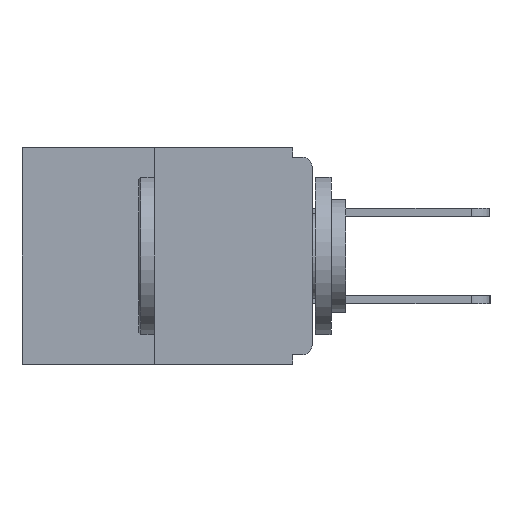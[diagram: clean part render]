
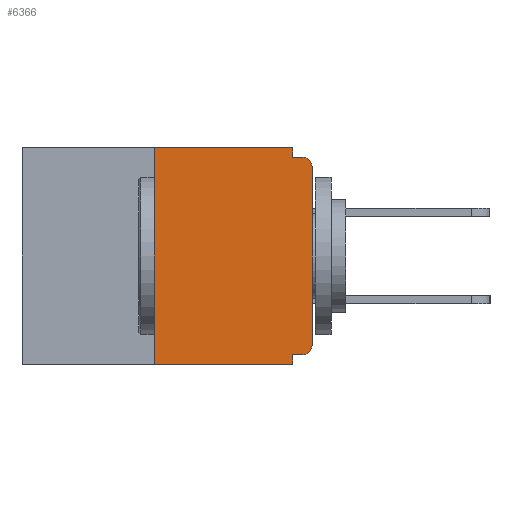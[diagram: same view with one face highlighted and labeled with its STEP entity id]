
A CAD part, left-side view. The second image highlights one B-rep face of the part: STEP entity #6366.
In plain terms, the highlighted planar face has unit normal (-1, 0, 0).
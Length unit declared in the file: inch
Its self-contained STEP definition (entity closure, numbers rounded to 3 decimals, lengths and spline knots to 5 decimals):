
#115 = VERTEX_POINT ( 'NONE', #15983 ) ;
#844 = LINE ( 'NONE', #16417, #10795 ) ;
#937 = EDGE_CURVE ( 'NONE', #18045, #11685, #17175, .T. ) ;
#1118 = EDGE_CURVE ( 'NONE', #1293, #15326, #21098, .T. ) ;
#1235 = DIRECTION ( 'NONE',  ( 0., 0., -1. ) ) ;
#1293 = VERTEX_POINT ( 'NONE', #21166 ) ;
#1443 = ORIENTED_EDGE ( 'NONE', *, *, #1118, .F. ) ;
#1468 = EDGE_CURVE ( 'NONE', #15326, #11685, #19242, .T. ) ;
#1549 = VECTOR ( 'NONE', #18733, 39.37008 ) ;
#1630 = CARTESIAN_POINT ( 'NONE',  ( 0., 0., -0.015 ) ) ;
#1633 = CARTESIAN_POINT ( 'NONE',  ( 0., 0., -0.03 ) ) ;
#2329 = CARTESIAN_POINT ( 'NONE',  ( 0., 0.031, -0.343 ) ) ;
#2448 = DIRECTION ( 'NONE',  ( 0., -1., 0. ) ) ;
#2455 = ORIENTED_EDGE ( 'NONE', *, *, #10482, .F. ) ;
#2511 = VECTOR ( 'NONE', #5447, 39.37008 ) ;
#2512 = EDGE_CURVE ( 'NONE', #3295, #115, #21164, .T. ) ;
#3079 = CARTESIAN_POINT ( 'NONE',  ( 0., 0.015, -0.313 ) ) ;
#3146 = DIRECTION ( 'NONE',  ( 0., 0., -1. ) ) ;
#3295 = VERTEX_POINT ( 'NONE', #12182 ) ;
#3360 = VERTEX_POINT ( 'NONE', #4072 ) ;
#3395 = ORIENTED_EDGE ( 'NONE', *, *, #15121, .F. ) ;
#3401 = VECTOR ( 'NONE', #2448, 39.37008 ) ;
#3425 = DIRECTION ( 'NONE',  ( 0., 0., 1. ) ) ;
#3602 = CARTESIAN_POINT ( 'NONE',  ( 0., 0., 0. ) ) ;
#4072 = CARTESIAN_POINT ( 'NONE',  ( 0., 0.031, -0.328 ) ) ;
#4421 = VECTOR ( 'NONE', #11365, 39.37008 ) ;
#4755 = LINE ( 'NONE', #20314, #6329 ) ;
#4812 = DIRECTION ( 'NONE',  ( -1., 0., 0. ) ) ;
#5447 = DIRECTION ( 'NONE',  ( 0., 0., 1. ) ) ;
#5563 = CARTESIAN_POINT ( 'NONE',  ( 0., 0.031, -0.015 ) ) ;
#5583 = VERTEX_POINT ( 'NONE', #19627 ) ;
#6329 = VECTOR ( 'NONE', #3425, 39.37008 ) ;
#6366 = ADVANCED_FACE ( 'NONE', ( #9306 ), #19575, .F. ) ;
#6676 = VERTEX_POINT ( 'NONE', #2329 ) ;
#6728 = VECTOR ( 'NONE', #8419, 39.37008 ) ;
#7259 = LINE ( 'NONE', #9906, #6728 ) ;
#8301 = CARTESIAN_POINT ( 'NONE',  ( 0., 0.031, -0.343 ) ) ;
#8419 = DIRECTION ( 'NONE',  ( 0., -1., 0. ) ) ;
#8740 = EDGE_LOOP ( 'NONE', ( #11450, #2455, #20168, #3395, #11189, #13838, #21576, #20918, #14046, #1443 ) ) ;
#8835 = CARTESIAN_POINT ( 'NONE',  ( 0., 0.25, 0. ) ) ;
#9253 = CARTESIAN_POINT ( 'NONE',  ( 0., 0.46, -0.343 ) ) ;
#9306 = FACE_OUTER_BOUND ( 'NONE', #8740, .T. ) ;
#9906 = CARTESIAN_POINT ( 'NONE',  ( 0., 0.46, 0. ) ) ;
#10482 = EDGE_CURVE ( 'NONE', #5583, #14031, #4755, .T. ) ;
#10747 = CARTESIAN_POINT ( 'NONE',  ( 0., 0.015, -0.03 ) ) ;
#10795 = VECTOR ( 'NONE', #20079, 39.37008 ) ;
#11189 = ORIENTED_EDGE ( 'NONE', *, *, #15161, .F. ) ;
#11365 = DIRECTION ( 'NONE',  ( 0., -1., 0. ) ) ;
#11450 = ORIENTED_EDGE ( 'NONE', *, *, #18557, .F. ) ;
#11685 = VERTEX_POINT ( 'NONE', #12885 ) ;
#12182 = CARTESIAN_POINT ( 'NONE',  ( 0., 0.015, -0.328 ) ) ;
#12885 = CARTESIAN_POINT ( 'NONE',  ( 0., 0.015, -0.015 ) ) ;
#13838 = ORIENTED_EDGE ( 'NONE', *, *, #2512, .T. ) ;
#14031 = VERTEX_POINT ( 'NONE', #8835 ) ;
#14046 = ORIENTED_EDGE ( 'NONE', *, *, #1468, .F. ) ;
#14277 = AXIS2_PLACEMENT_3D ( 'NONE', #3079, #19758, #3146 ) ;
#15121 = EDGE_CURVE ( 'NONE', #3360, #6676, #20641, .T. ) ;
#15161 = EDGE_CURVE ( 'NONE', #3295, #3360, #844, .T. ) ;
#15326 = VERTEX_POINT ( 'NONE', #5563 ) ;
#15983 = CARTESIAN_POINT ( 'NONE',  ( 0., 0., -0.313 ) ) ;
#16300 = LINE ( 'NONE', #3602, #2511 ) ;
#16312 = EDGE_CURVE ( 'NONE', #5583, #6676, #19798, .T. ) ;
#16417 = CARTESIAN_POINT ( 'NONE',  ( 0., 0., -0.328 ) ) ;
#17175 = CIRCLE ( 'NONE', #18149, 0.015 ) ;
#18045 = VERTEX_POINT ( 'NONE', #1633 ) ;
#18149 = AXIS2_PLACEMENT_3D ( 'NONE', #10747, #4812, #19718 ) ;
#18164 = DIRECTION ( 'NONE',  ( 0., 0., -1. ) ) ;
#18557 = EDGE_CURVE ( 'NONE', #14031, #1293, #7259, .T. ) ;
#18588 = CARTESIAN_POINT ( 'NONE',  ( 0., 0.031, 0. ) ) ;
#18733 = DIRECTION ( 'NONE',  ( 0., 0., -1. ) ) ;
#18895 = AXIS2_PLACEMENT_3D ( 'NONE', #19436, #21123, #1235 ) ;
#19057 = VECTOR ( 'NONE', #18164, 39.37008 ) ;
#19242 = LINE ( 'NONE', #1630, #4421 ) ;
#19331 = EDGE_CURVE ( 'NONE', #115, #18045, #16300, .T. ) ;
#19436 = CARTESIAN_POINT ( 'NONE',  ( 0., 0.46, 0. ) ) ;
#19575 = PLANE ( 'NONE',  #18895 ) ;
#19627 = CARTESIAN_POINT ( 'NONE',  ( 0., 0.25, -0.343 ) ) ;
#19718 = DIRECTION ( 'NONE',  ( 0., 0., -1. ) ) ;
#19758 = DIRECTION ( 'NONE',  ( -1., 0., 0. ) ) ;
#19798 = LINE ( 'NONE', #9253, #3401 ) ;
#20079 = DIRECTION ( 'NONE',  ( 0., 1., 0. ) ) ;
#20168 = ORIENTED_EDGE ( 'NONE', *, *, #16312, .T. ) ;
#20314 = CARTESIAN_POINT ( 'NONE',  ( 0., 0.25, 0. ) ) ;
#20641 = LINE ( 'NONE', #8301, #19057 ) ;
#20918 = ORIENTED_EDGE ( 'NONE', *, *, #937, .T. ) ;
#21098 = LINE ( 'NONE', #18588, #1549 ) ;
#21123 = DIRECTION ( 'NONE',  ( 1., 0., 0. ) ) ;
#21164 = CIRCLE ( 'NONE', #14277, 0.015 ) ;
#21166 = CARTESIAN_POINT ( 'NONE',  ( 0., 0.031, 0. ) ) ;
#21576 = ORIENTED_EDGE ( 'NONE', *, *, #19331, .T. ) ;
